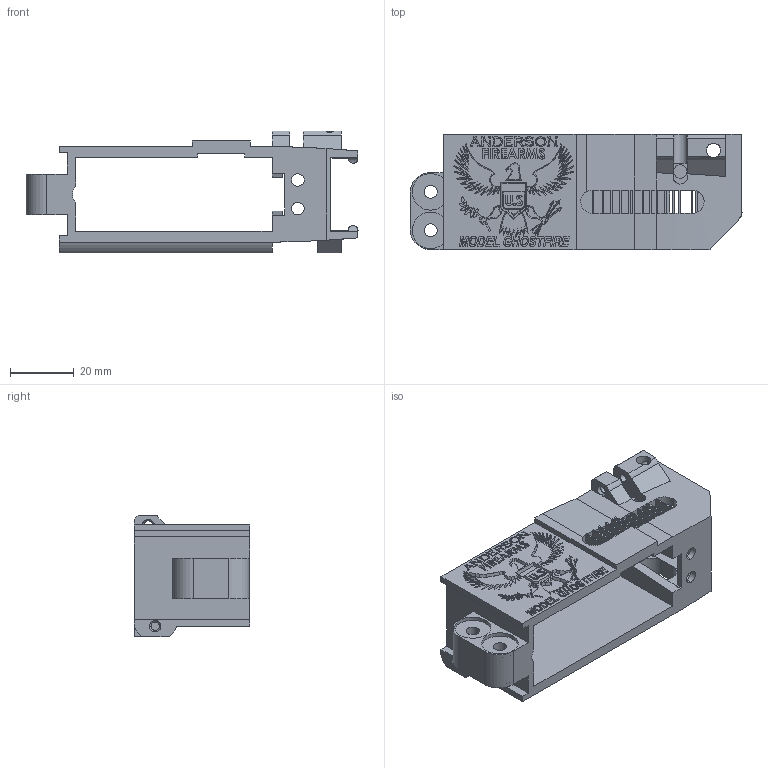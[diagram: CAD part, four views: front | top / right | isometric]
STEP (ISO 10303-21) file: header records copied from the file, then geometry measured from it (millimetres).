
FILE_DESCRIPTION (( 'STEP AP203' ), '1' );
FILE_NAME ('MagazineWell.STEP', '2019-09-03T07:05:17', ( '' ), ( '' ), 'SwSTEP 2.0', 'SolidWorks 2018', '' );
FILE_SCHEMA (( 'CONFIG_CONTROL_DESIGN' ));
Products named in the file (1): MagazineWell
Bounding box: 104.19 x 36.15 x 38.28 mm (x, y, z)
Volume: 31157.8 mm3; surface area: 24327.9 mm2
Topology: 1 solids, 1 shells, 2471 faces, 6810 edges, 4509 vertices
Faces by surface type: plane 1732, bspline 642, cylinder 86, cone 11
Entity records: 110365 total; most frequent: CARTESIAN_POINT 51638, ORIENTED_EDGE 13620, DIRECTION 9296, EDGE_CURVE 6810, VECTOR 5268, LINE 5268, VERTEX_POINT 4509, EDGE_LOOP 2701
